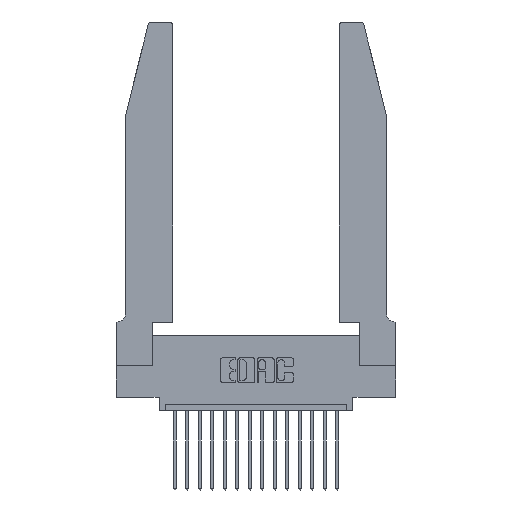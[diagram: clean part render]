
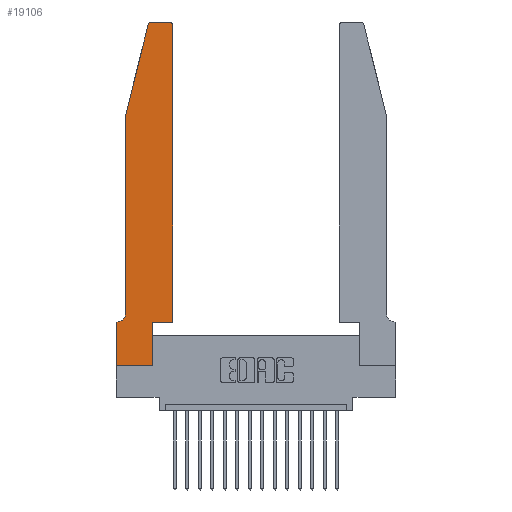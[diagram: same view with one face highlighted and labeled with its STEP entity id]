
A CAD part, top view. The second image highlights one B-rep face of the part: STEP entity #19106.
In plain terms, the highlighted planar face has unit normal (0, 0, 1).
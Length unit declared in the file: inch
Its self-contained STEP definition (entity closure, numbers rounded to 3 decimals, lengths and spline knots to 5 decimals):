
#95 = EDGE_CURVE ( 'NONE', #17417, #8420, #1017, .T. ) ;
#187 = VERTEX_POINT ( 'NONE', #12717 ) ;
#775 = VERTEX_POINT ( 'NONE', #8421 ) ;
#810 = DIRECTION ( 'NONE',  ( -1., 0., 0. ) ) ;
#905 = LINE ( 'NONE', #15093, #13666 ) ;
#1017 = LINE ( 'NONE', #8062, #18203 ) ;
#1061 = CARTESIAN_POINT ( 'NONE',  ( 0.4505, 0.35, 0.37 ) ) ;
#1101 = CARTESIAN_POINT ( 'NONE',  ( 0.0755, 0.42, 0.37 ) ) ;
#1137 = CARTESIAN_POINT ( 'NONE',  ( 0.284, 2.75, 0.37 ) ) ;
#1160 = DIRECTION ( 'NONE',  ( 1., 0., 0. ) ) ;
#1533 = LINE ( 'NONE', #7118, #6123 ) ;
#1717 = CARTESIAN_POINT ( 'NONE',  ( 0., 0., 0.37 ) ) ;
#2122 = CARTESIAN_POINT ( 'NONE',  ( 0., 0.35, 0.37 ) ) ;
#2592 = CARTESIAN_POINT ( 'NONE',  ( 0.25487, 2.72718, 0.37 ) ) ;
#2667 = CARTESIAN_POINT ( 'NONE',  ( 0.284, 2.72, 0.37 ) ) ;
#2757 = VERTEX_POINT ( 'NONE', #1137 ) ;
#3156 = AXIS2_PLACEMENT_3D ( 'NONE', #2667, #4216, #17154 ) ;
#3264 = DIRECTION ( 'NONE',  ( 0., -1., 0. ) ) ;
#3309 = EDGE_CURVE ( 'NONE', #5488, #10491, #3691, .T. ) ;
#3691 = LINE ( 'NONE', #10774, #15724 ) ;
#4180 = EDGE_CURVE ( 'NONE', #187, #775, #14298, .T. ) ;
#4216 = DIRECTION ( 'NONE',  ( 0., 0., 1. ) ) ;
#4292 = VERTEX_POINT ( 'NONE', #1101 ) ;
#4309 = CARTESIAN_POINT ( 'NONE',  ( 0.4205, 2.75, 0.37 ) ) ;
#4776 = EDGE_CURVE ( 'NONE', #10665, #10314, #17552, .T. ) ;
#4903 = EDGE_CURVE ( 'NONE', #8420, #4292, #5717, .T. ) ;
#5488 = VERTEX_POINT ( 'NONE', #1061 ) ;
#5545 = DIRECTION ( 'NONE',  ( 1., 0., 0. ) ) ;
#5717 = LINE ( 'NONE', #6983, #11744 ) ;
#6004 = VECTOR ( 'NONE', #14893, 39.37008 ) ;
#6100 = CARTESIAN_POINT ( 'NONE',  ( 0.4505, 2.72, 0.37 ) ) ;
#6123 = VECTOR ( 'NONE', #1160, 39.37008 ) ;
#6713 = DIRECTION ( 'NONE',  ( -0.239, -0.971, 0. ) ) ;
#6935 = CIRCLE ( 'NONE', #12303, 0.07 ) ;
#6961 = EDGE_LOOP ( 'NONE', ( #10102, #16393, #15152, #9645, #18035, #16600, #13261, #7766, #17315, #7222, #11236, #11161 ) ) ;
#6983 = CARTESIAN_POINT ( 'NONE',  ( 0.0755, 2., 0.37 ) ) ;
#7064 = CARTESIAN_POINT ( 'NONE',  ( 0.4205, 2.72, 0.37 ) ) ;
#7118 = CARTESIAN_POINT ( 'NONE',  ( 0.4505, 0.35, 0.37 ) ) ;
#7222 = ORIENTED_EDGE ( 'NONE', *, *, #9302, .T. ) ;
#7306 = VECTOR ( 'NONE', #3264, 39.37008 ) ;
#7550 = EDGE_CURVE ( 'NONE', #10314, #187, #10810, .T. ) ;
#7766 = ORIENTED_EDGE ( 'NONE', *, *, #4180, .T. ) ;
#7873 = CIRCLE ( 'NONE', #3156, 0.03 ) ;
#7924 = CARTESIAN_POINT ( 'NONE',  ( 0.0055, 0.35, 0.37 ) ) ;
#8062 = CARTESIAN_POINT ( 'NONE',  ( 0.0755, 2., 0.37 ) ) ;
#8108 = PLANE ( 'NONE',  #8690 ) ;
#8334 = EDGE_CURVE ( 'NONE', #10491, #18120, #13585, .T. ) ;
#8420 = VERTEX_POINT ( 'NONE', #11697 ) ;
#8421 = CARTESIAN_POINT ( 'NONE',  ( 0.2865, 0., 0.37 ) ) ;
#8690 = AXIS2_PLACEMENT_3D ( 'NONE', #2122, #11048, #16841 ) ;
#9130 = CARTESIAN_POINT ( 'NONE',  ( 0.0055, 0.42, 0.37 ) ) ;
#9213 = CARTESIAN_POINT ( 'NONE',  ( 0.2865, 0.35, 0.37 ) ) ;
#9302 = EDGE_CURVE ( 'NONE', #16127, #5488, #1533, .T. ) ;
#9645 = ORIENTED_EDGE ( 'NONE', *, *, #4903, .T. ) ;
#10102 = ORIENTED_EDGE ( 'NONE', *, *, #18840, .T. ) ;
#10314 = VERTEX_POINT ( 'NONE', #12543 ) ;
#10491 = VERTEX_POINT ( 'NONE', #6100 ) ;
#10665 = VERTEX_POINT ( 'NONE', #7924 ) ;
#10774 = CARTESIAN_POINT ( 'NONE',  ( 0.4505, 0.35, 0.37 ) ) ;
#10810 = LINE ( 'NONE', #1717, #7306 ) ;
#11042 = EDGE_CURVE ( 'NONE', #2757, #17417, #7873, .T. ) ;
#11048 = DIRECTION ( 'NONE',  ( 0., 0., 1. ) ) ;
#11161 = ORIENTED_EDGE ( 'NONE', *, *, #8334, .T. ) ;
#11236 = ORIENTED_EDGE ( 'NONE', *, *, #3309, .T. ) ;
#11697 = CARTESIAN_POINT ( 'NONE',  ( 0.0755, 2., 0.37 ) ) ;
#11744 = VECTOR ( 'NONE', #16012, 39.37008 ) ;
#12303 = AXIS2_PLACEMENT_3D ( 'NONE', #9130, #14829, #15025 ) ;
#12543 = CARTESIAN_POINT ( 'NONE',  ( 0., 0.35, 0.37 ) ) ;
#12602 = CARTESIAN_POINT ( 'NONE',  ( 0.0755, 0.35, 0.37 ) ) ;
#12717 = CARTESIAN_POINT ( 'NONE',  ( 0., 0., 0.37 ) ) ;
#12958 = DIRECTION ( 'NONE',  ( 1., 0., 0. ) ) ;
#13075 = DIRECTION ( 'NONE',  ( 0., 0., 1. ) ) ;
#13226 = LINE ( 'NONE', #13434, #6004 ) ;
#13261 = ORIENTED_EDGE ( 'NONE', *, *, #7550, .T. ) ;
#13434 = CARTESIAN_POINT ( 'NONE',  ( 0.2605, 2.75, 0.37 ) ) ;
#13585 = CIRCLE ( 'NONE', #13679, 0.03 ) ;
#13666 = VECTOR ( 'NONE', #18124, 39.37008 ) ;
#13679 = AXIS2_PLACEMENT_3D ( 'NONE', #7064, #13075, #5545 ) ;
#14270 = VECTOR ( 'NONE', #810, 39.37008 ) ;
#14298 = LINE ( 'NONE', #15971, #18986 ) ;
#14829 = DIRECTION ( 'NONE',  ( 0., 0., -1. ) ) ;
#14893 = DIRECTION ( 'NONE',  ( -1., 0., 0. ) ) ;
#15025 = DIRECTION ( 'NONE',  ( -1., 0., 0. ) ) ;
#15093 = CARTESIAN_POINT ( 'NONE',  ( 0.2865, 0.35, 0.37 ) ) ;
#15105 = DIRECTION ( 'NONE',  ( 0., 1., 0. ) ) ;
#15152 = ORIENTED_EDGE ( 'NONE', *, *, #95, .T. ) ;
#15248 = FACE_OUTER_BOUND ( 'NONE', #6961, .T. ) ;
#15724 = VECTOR ( 'NONE', #15105, 39.37008 ) ;
#15971 = CARTESIAN_POINT ( 'NONE',  ( 0., 0., 0.37 ) ) ;
#16012 = DIRECTION ( 'NONE',  ( 0., -1., 0. ) ) ;
#16127 = VERTEX_POINT ( 'NONE', #9213 ) ;
#16393 = ORIENTED_EDGE ( 'NONE', *, *, #11042, .T. ) ;
#16600 = ORIENTED_EDGE ( 'NONE', *, *, #4776, .T. ) ;
#16841 = DIRECTION ( 'NONE',  ( 1., 0., 0. ) ) ;
#17031 = EDGE_CURVE ( 'NONE', #4292, #10665, #6935, .T. ) ;
#17154 = DIRECTION ( 'NONE',  ( 1., 0., 0. ) ) ;
#17315 = ORIENTED_EDGE ( 'NONE', *, *, #18989, .T. ) ;
#17417 = VERTEX_POINT ( 'NONE', #2592 ) ;
#17552 = LINE ( 'NONE', #12602, #14270 ) ;
#18035 = ORIENTED_EDGE ( 'NONE', *, *, #17031, .T. ) ;
#18120 = VERTEX_POINT ( 'NONE', #4309 ) ;
#18124 = DIRECTION ( 'NONE',  ( 0., 1., 0. ) ) ;
#18203 = VECTOR ( 'NONE', #6713, 39.37008 ) ;
#18840 = EDGE_CURVE ( 'NONE', #18120, #2757, #13226, .T. ) ;
#18986 = VECTOR ( 'NONE', #12958, 39.37008 ) ;
#18989 = EDGE_CURVE ( 'NONE', #775, #16127, #905, .T. ) ;
#19106 = ADVANCED_FACE ( 'NONE', ( #15248 ), #8108, .T. ) ;
